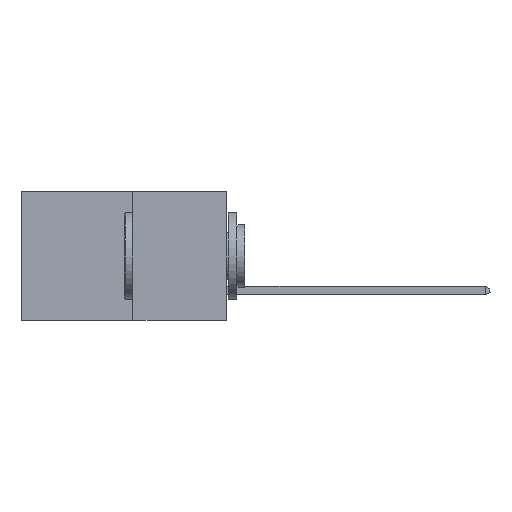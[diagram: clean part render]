
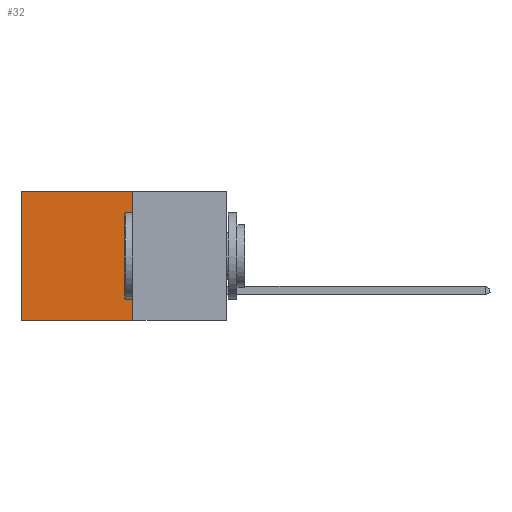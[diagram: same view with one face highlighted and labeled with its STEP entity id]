
A CAD part, left-side view. The second image highlights one B-rep face of the part: STEP entity #32.
In plain terms, the highlighted planar face has unit normal (-1, 0, 0).
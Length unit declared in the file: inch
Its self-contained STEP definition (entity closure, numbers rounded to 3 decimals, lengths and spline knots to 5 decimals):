
#32 = ADVANCED_FACE ( 'NONE', ( #10226 ), #16916, .F. ) ;
#151 = CARTESIAN_POINT ( 'NONE',  ( 0.277, 0.27, 0. ) ) ;
#272 = DIRECTION ( 'NONE',  ( 0., 0., -1. ) ) ;
#300 = DIRECTION ( 'NONE',  ( 1., 0., 0. ) ) ;
#994 = LINE ( 'NONE', #14275, #4218 ) ;
#1350 = VERTEX_POINT ( 'NONE', #9853 ) ;
#1985 = EDGE_CURVE ( 'NONE', #1350, #15652, #994, .T. ) ;
#2299 = CARTESIAN_POINT ( 'NONE',  ( 0.277, 0.27, 0. ) ) ;
#3222 = ORIENTED_EDGE ( 'NONE', *, *, #18872, .T. ) ;
#3313 = VECTOR ( 'NONE', #12890, 39.37008 ) ;
#3386 = CARTESIAN_POINT ( 'NONE',  ( 0.277, 0.59, -0.37 ) ) ;
#3828 = LINE ( 'NONE', #11322, #3313 ) ;
#4131 = EDGE_CURVE ( 'NONE', #19212, #15652, #5327, .T. ) ;
#4147 = VECTOR ( 'NONE', #11788, 39.37008 ) ;
#4218 = VECTOR ( 'NONE', #13613, 39.37008 ) ;
#5239 = AXIS2_PLACEMENT_3D ( 'NONE', #12689, #300, #272 ) ;
#5327 = LINE ( 'NONE', #14886, #16857 ) ;
#5569 = EDGE_LOOP ( 'NONE', ( #17224, #11931, #17978, #3222 ) ) ;
#8349 = LINE ( 'NONE', #2299, #4147 ) ;
#9853 = CARTESIAN_POINT ( 'NONE',  ( 0.277, 0.59, 0. ) ) ;
#10226 = FACE_OUTER_BOUND ( 'NONE', #5569, .T. ) ;
#11204 = CARTESIAN_POINT ( 'NONE',  ( 0.277, 0.27, -0.37 ) ) ;
#11322 = CARTESIAN_POINT ( 'NONE',  ( 0.277, 0.27, -0.37 ) ) ;
#11552 = VERTEX_POINT ( 'NONE', #151 ) ;
#11788 = DIRECTION ( 'NONE',  ( 0., 1., 0. ) ) ;
#11931 = ORIENTED_EDGE ( 'NONE', *, *, #4131, .F. ) ;
#12689 = CARTESIAN_POINT ( 'NONE',  ( 0.277, 0.27, -0.37 ) ) ;
#12890 = DIRECTION ( 'NONE',  ( 0., 0., -1. ) ) ;
#13613 = DIRECTION ( 'NONE',  ( 0., 0., -1. ) ) ;
#14275 = CARTESIAN_POINT ( 'NONE',  ( 0.277, 0.59, -0.37 ) ) ;
#14780 = DIRECTION ( 'NONE',  ( 0., 1., 0. ) ) ;
#14886 = CARTESIAN_POINT ( 'NONE',  ( 0.277, 0.27, -0.37 ) ) ;
#15013 = EDGE_CURVE ( 'NONE', #11552, #19212, #3828, .T. ) ;
#15652 = VERTEX_POINT ( 'NONE', #3386 ) ;
#16857 = VECTOR ( 'NONE', #14780, 39.37008 ) ;
#16916 = PLANE ( 'NONE',  #5239 ) ;
#17224 = ORIENTED_EDGE ( 'NONE', *, *, #1985, .T. ) ;
#17978 = ORIENTED_EDGE ( 'NONE', *, *, #15013, .F. ) ;
#18872 = EDGE_CURVE ( 'NONE', #11552, #1350, #8349, .T. ) ;
#19212 = VERTEX_POINT ( 'NONE', #11204 ) ;
